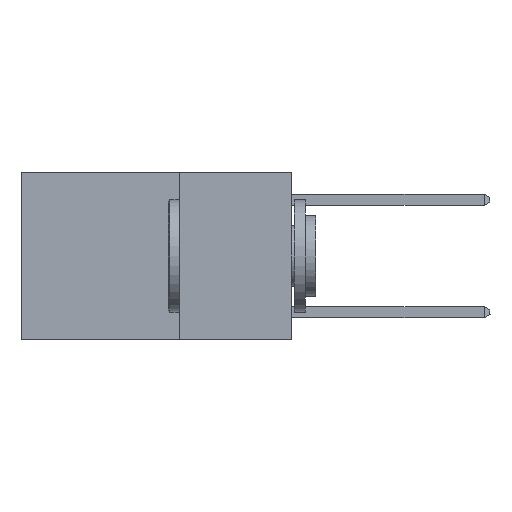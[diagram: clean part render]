
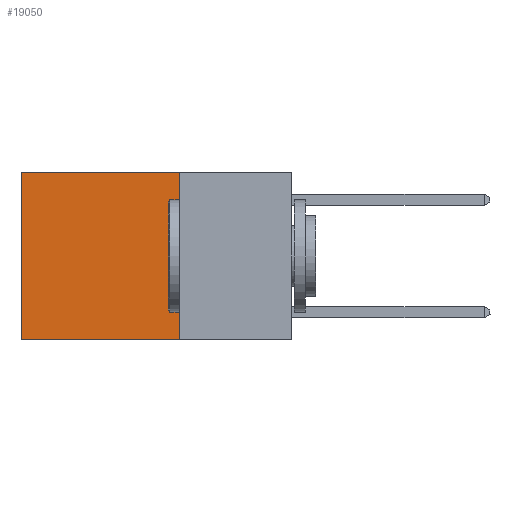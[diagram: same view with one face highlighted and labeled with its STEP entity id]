
A CAD part, left-side view. The second image highlights one B-rep face of the part: STEP entity #19050.
In plain terms, the highlighted planar face has unit normal (-1, 0, 0).
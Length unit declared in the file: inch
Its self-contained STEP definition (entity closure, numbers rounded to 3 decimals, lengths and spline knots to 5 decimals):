
#1648 = VERTEX_POINT ( 'NONE', #11700 ) ;
#1751 = EDGE_CURVE ( 'NONE', #5570, #11257, #15517, .T. ) ;
#3321 = CARTESIAN_POINT ( 'NONE',  ( 0.2625, 0.25, 0. ) ) ;
#3957 = DIRECTION ( 'NONE',  ( 0., 1., 0. ) ) ;
#5570 = VERTEX_POINT ( 'NONE', #17040 ) ;
#5984 = ORIENTED_EDGE ( 'NONE', *, *, #1751, .T. ) ;
#6219 = ORIENTED_EDGE ( 'NONE', *, *, #14789, .F. ) ;
#6366 = LINE ( 'NONE', #16811, #22092 ) ;
#6849 = EDGE_CURVE ( 'NONE', #1648, #5570, #9047, .T. ) ;
#6873 = ORIENTED_EDGE ( 'NONE', *, *, #15647, .F. ) ;
#7152 = CARTESIAN_POINT ( 'NONE',  ( 0.2625, 0.25, -0.37 ) ) ;
#7198 = ORIENTED_EDGE ( 'NONE', *, *, #6849, .T. ) ;
#7332 = PLANE ( 'NONE',  #14435 ) ;
#7402 = VECTOR ( 'NONE', #3957, 39.37008 ) ;
#9047 = LINE ( 'NONE', #3321, #19149 ) ;
#11257 = VERTEX_POINT ( 'NONE', #22559 ) ;
#11700 = CARTESIAN_POINT ( 'NONE',  ( 0.2625, 0.25, 0. ) ) ;
#11881 = VERTEX_POINT ( 'NONE', #7152 ) ;
#12107 = CARTESIAN_POINT ( 'NONE',  ( 0.2625, 0.6, 0. ) ) ;
#13155 = LINE ( 'NONE', #13902, #7402 ) ;
#13191 = DIRECTION ( 'NONE',  ( 0., 0., -1. ) ) ;
#13354 = DIRECTION ( 'NONE',  ( 0., 1., 0. ) ) ;
#13902 = CARTESIAN_POINT ( 'NONE',  ( 0.2625, 0.25, -0.37 ) ) ;
#14435 = AXIS2_PLACEMENT_3D ( 'NONE', #20590, #24155, #13191 ) ;
#14789 = EDGE_CURVE ( 'NONE', #11881, #11257, #13155, .T. ) ;
#15513 = VECTOR ( 'NONE', #17784, 39.37008 ) ;
#15517 = LINE ( 'NONE', #12107, #15513 ) ;
#15647 = EDGE_CURVE ( 'NONE', #1648, #11881, #6366, .T. ) ;
#16811 = CARTESIAN_POINT ( 'NONE',  ( 0.2625, 0.25, 0. ) ) ;
#17040 = CARTESIAN_POINT ( 'NONE',  ( 0.2625, 0.6, 0. ) ) ;
#17784 = DIRECTION ( 'NONE',  ( 0., 0., -1. ) ) ;
#17973 = FACE_OUTER_BOUND ( 'NONE', #18683, .T. ) ;
#18612 = DIRECTION ( 'NONE',  ( 0., 0., -1. ) ) ;
#18683 = EDGE_LOOP ( 'NONE', ( #5984, #6219, #6873, #7198 ) ) ;
#19050 = ADVANCED_FACE ( 'NONE', ( #17973 ), #7332, .F. ) ;
#19149 = VECTOR ( 'NONE', #13354, 39.37008 ) ;
#20590 = CARTESIAN_POINT ( 'NONE',  ( 0.2625, 0.25, 0. ) ) ;
#22092 = VECTOR ( 'NONE', #18612, 39.37008 ) ;
#22559 = CARTESIAN_POINT ( 'NONE',  ( 0.2625, 0.6, -0.37 ) ) ;
#24155 = DIRECTION ( 'NONE',  ( 1., 0., 0. ) ) ;
